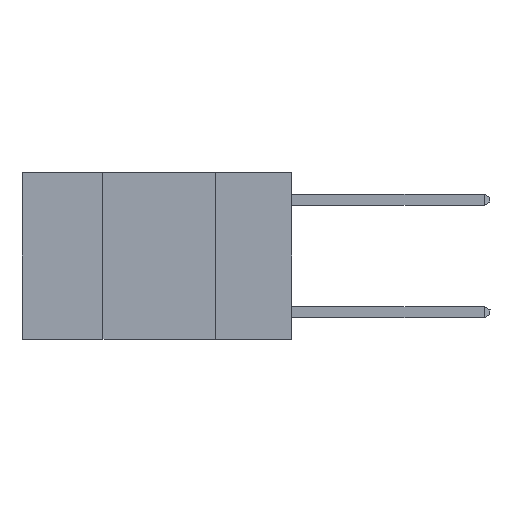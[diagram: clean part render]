
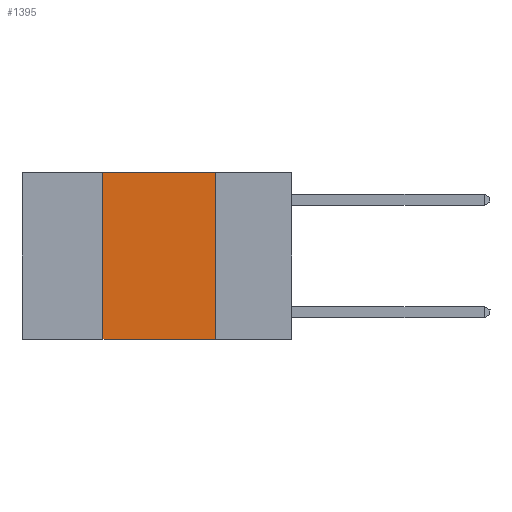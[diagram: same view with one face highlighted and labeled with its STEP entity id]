
A CAD part, left-side view. The second image highlights one B-rep face of the part: STEP entity #1395.
In plain terms, the highlighted planar face has unit normal (-1, 0, 0).
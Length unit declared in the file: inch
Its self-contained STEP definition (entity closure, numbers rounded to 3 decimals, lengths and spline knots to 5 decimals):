
#261 = CARTESIAN_POINT ( 'NONE',  ( 0., 0.6, 0. ) ) ;
#1147 = EDGE_LOOP ( 'NONE', ( #22124, #22842, #23063, #23125 ) ) ;
#1395 = ADVANCED_FACE ( 'NONE', ( #12268 ), #24548, .F. ) ;
#1400 = CARTESIAN_POINT ( 'NONE',  ( 0., 0.6, 0. ) ) ;
#1801 = CARTESIAN_POINT ( 'NONE',  ( 0., 0.17, 0. ) ) ;
#3973 = DIRECTION ( 'NONE',  ( 0., 0., -1. ) ) ;
#6531 = VECTOR ( 'NONE', #29860, 39.37008 ) ;
#7633 = CARTESIAN_POINT ( 'NONE',  ( 0., 0.42, -0.37 ) ) ;
#7780 = AXIS2_PLACEMENT_3D ( 'NONE', #261, #26950, #12553 ) ;
#10165 = DIRECTION ( 'NONE',  ( 0., -1., 0. ) ) ;
#11362 = VERTEX_POINT ( 'NONE', #14439 ) ;
#12079 = CARTESIAN_POINT ( 'NONE',  ( 0., 0.17, -0.37 ) ) ;
#12268 = FACE_OUTER_BOUND ( 'NONE', #1147, .T. ) ;
#12553 = DIRECTION ( 'NONE',  ( 0., 0., -1. ) ) ;
#12613 = VERTEX_POINT ( 'NONE', #12079 ) ;
#14439 = CARTESIAN_POINT ( 'NONE',  ( 0., 0.17, 0. ) ) ;
#15092 = VERTEX_POINT ( 'NONE', #7633 ) ;
#15939 = VERTEX_POINT ( 'NONE', #25053 ) ;
#17181 = VECTOR ( 'NONE', #3973, 39.37008 ) ;
#18630 = EDGE_CURVE ( 'NONE', #15939, #11362, #25660, .T. ) ;
#19272 = VECTOR ( 'NONE', #20784, 39.37008 ) ;
#20784 = DIRECTION ( 'NONE',  ( 0., -1., 0. ) ) ;
#22124 = ORIENTED_EDGE ( 'NONE', *, *, #23235, .F. ) ;
#22842 = ORIENTED_EDGE ( 'NONE', *, *, #18630, .F. ) ;
#23063 = ORIENTED_EDGE ( 'NONE', *, *, #28027, .F. ) ;
#23125 = ORIENTED_EDGE ( 'NONE', *, *, #29621, .T. ) ;
#23235 = EDGE_CURVE ( 'NONE', #11362, #12613, #30599, .T. ) ;
#24533 = VECTOR ( 'NONE', #10165, 39.37008 ) ;
#24548 = PLANE ( 'NONE',  #7780 ) ;
#25053 = CARTESIAN_POINT ( 'NONE',  ( 0., 0.42, 0. ) ) ;
#25258 = LINE ( 'NONE', #26877, #24533 ) ;
#25660 = LINE ( 'NONE', #1400, #19272 ) ;
#25755 = LINE ( 'NONE', #27480, #6531 ) ;
#26877 = CARTESIAN_POINT ( 'NONE',  ( 0., 0.6, -0.37 ) ) ;
#26950 = DIRECTION ( 'NONE',  ( 1., 0., 0. ) ) ;
#27480 = CARTESIAN_POINT ( 'NONE',  ( 0., 0.42, 0. ) ) ;
#28027 = EDGE_CURVE ( 'NONE', #15092, #15939, #25755, .T. ) ;
#29621 = EDGE_CURVE ( 'NONE', #15092, #12613, #25258, .T. ) ;
#29860 = DIRECTION ( 'NONE',  ( 0., 0., 1. ) ) ;
#30599 = LINE ( 'NONE', #1801, #17181 ) ;
